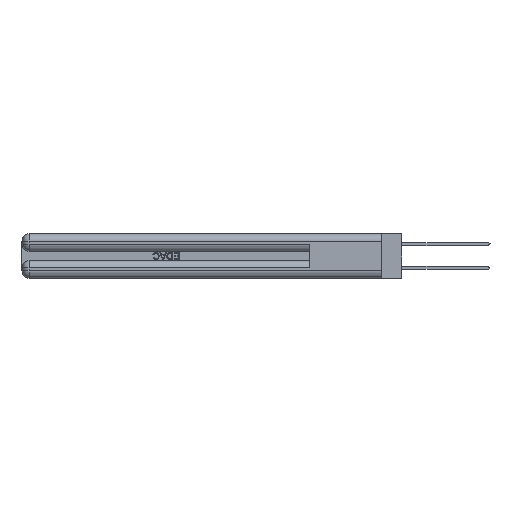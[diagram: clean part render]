
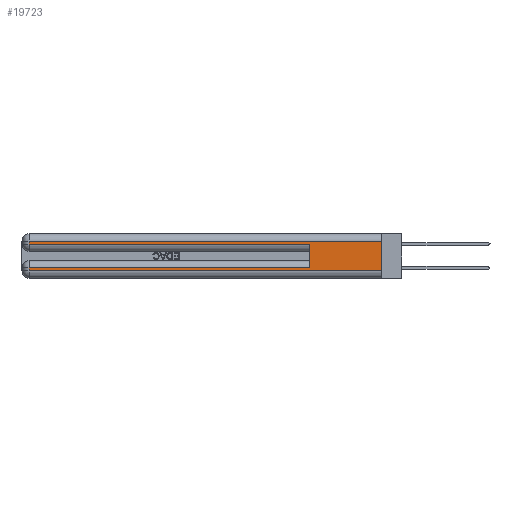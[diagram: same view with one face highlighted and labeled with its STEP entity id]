
A CAD part, left-side view. The second image highlights one B-rep face of the part: STEP entity #19723.
In plain terms, the highlighted planar face has unit normal (-1, 0, 0).
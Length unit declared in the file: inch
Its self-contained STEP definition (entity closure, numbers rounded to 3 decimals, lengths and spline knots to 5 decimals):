
#172 = EDGE_CURVE ( 'NONE', #41461, #45304, #2076, .T. ) ;
#293 = CARTESIAN_POINT ( 'NONE',  ( 0., 0., 0.085 ) ) ;
#947 = CARTESIAN_POINT ( 'NONE',  ( 0., 0., 0.37 ) ) ;
#2076 = LINE ( 'NONE', #7355, #39697 ) ;
#2754 = LINE ( 'NONE', #13703, #36304 ) ;
#3650 = LINE ( 'NONE', #4636, #18855 ) ;
#4143 = CARTESIAN_POINT ( 'NONE',  ( 0., 2.94, 0.31 ) ) ;
#4265 = CARTESIAN_POINT ( 'NONE',  ( 0., 2.94, 0.06 ) ) ;
#4636 = CARTESIAN_POINT ( 'NONE',  ( 0., 2.94, 0.37 ) ) ;
#5102 = CARTESIAN_POINT ( 'NONE',  ( 0., 0., 0.31 ) ) ;
#5394 = ORIENTED_EDGE ( 'NONE', *, *, #16337, .T. ) ;
#5699 = LINE ( 'NONE', #9321, #15059 ) ;
#6045 = DIRECTION ( 'NONE',  ( 0., -1., 0. ) ) ;
#6393 = PLANE ( 'NONE',  #37732 ) ;
#7355 = CARTESIAN_POINT ( 'NONE',  ( 0., 2.94, 0.37 ) ) ;
#8969 = VECTOR ( 'NONE', #22757, 39.37008 ) ;
#9321 = CARTESIAN_POINT ( 'NONE',  ( 0., 0., 0.06 ) ) ;
#10417 = EDGE_CURVE ( 'NONE', #42172, #28726, #33186, .T. ) ;
#11933 = VECTOR ( 'NONE', #39482, 39.37008 ) ;
#12002 = DIRECTION ( 'NONE',  ( 0., 0., -1. ) ) ;
#13620 = EDGE_CURVE ( 'NONE', #42172, #26062, #44048, .T. ) ;
#13703 = CARTESIAN_POINT ( 'NONE',  ( 0., 0.6, 0.145 ) ) ;
#15059 = VECTOR ( 'NONE', #6045, 39.37008 ) ;
#15963 = CARTESIAN_POINT ( 'NONE',  ( 0., 0.6, 0.085 ) ) ;
#16337 = EDGE_CURVE ( 'NONE', #29624, #45047, #26652, .T. ) ;
#16600 = CARTESIAN_POINT ( 'NONE',  ( 0., 0., 0.31 ) ) ;
#16651 = DIRECTION ( 'NONE',  ( 0., 0., -1. ) ) ;
#17339 = DIRECTION ( 'NONE',  ( 1., 0., 0. ) ) ;
#18855 = VECTOR ( 'NONE', #12002, 39.37008 ) ;
#19723 = ADVANCED_FACE ( 'NONE', ( #25156 ), #6393, .F. ) ;
#21315 = CARTESIAN_POINT ( 'NONE',  ( 0., 0., 0.37 ) ) ;
#21465 = ORIENTED_EDGE ( 'NONE', *, *, #13620, .T. ) ;
#22361 = EDGE_LOOP ( 'NONE', ( #28012, #21465, #35559, #5394, #24233, #41038, #42004, #28893 ) ) ;
#22757 = DIRECTION ( 'NONE',  ( 0., 1., 0. ) ) ;
#23134 = EDGE_CURVE ( 'NONE', #32164, #41461, #41915, .T. ) ;
#24019 = DIRECTION ( 'NONE',  ( 0., 1., 0. ) ) ;
#24233 = ORIENTED_EDGE ( 'NONE', *, *, #48264, .F. ) ;
#24328 = CARTESIAN_POINT ( 'NONE',  ( 0., 0., 0.285 ) ) ;
#25156 = FACE_OUTER_BOUND ( 'NONE', #22361, .T. ) ;
#26062 = VERTEX_POINT ( 'NONE', #4143 ) ;
#26652 = LINE ( 'NONE', #24328, #11933 ) ;
#28012 = ORIENTED_EDGE ( 'NONE', *, *, #10417, .F. ) ;
#28726 = VERTEX_POINT ( 'NONE', #34109 ) ;
#28893 = ORIENTED_EDGE ( 'NONE', *, *, #33861, .T. ) ;
#29624 = VERTEX_POINT ( 'NONE', #36515 ) ;
#32164 = VERTEX_POINT ( 'NONE', #15963 ) ;
#33186 = LINE ( 'NONE', #947, #37291 ) ;
#33861 = EDGE_CURVE ( 'NONE', #45304, #28726, #5699, .T. ) ;
#34030 = VECTOR ( 'NONE', #24019, 39.37008 ) ;
#34109 = CARTESIAN_POINT ( 'NONE',  ( 0., 0., 0.06 ) ) ;
#35553 = CARTESIAN_POINT ( 'NONE',  ( 0., 0.6, 0.285 ) ) ;
#35559 = ORIENTED_EDGE ( 'NONE', *, *, #44638, .T. ) ;
#36304 = VECTOR ( 'NONE', #39059, 39.37008 ) ;
#36326 = DIRECTION ( 'NONE',  ( 0., 0., -1. ) ) ;
#36515 = CARTESIAN_POINT ( 'NONE',  ( 0., 2.94, 0.285 ) ) ;
#37291 = VECTOR ( 'NONE', #16651, 39.37008 ) ;
#37732 = AXIS2_PLACEMENT_3D ( 'NONE', #21315, #17339, #36326 ) ;
#39059 = DIRECTION ( 'NONE',  ( 0., 0., 1. ) ) ;
#39482 = DIRECTION ( 'NONE',  ( 0., -1., 0. ) ) ;
#39697 = VECTOR ( 'NONE', #48184, 39.37008 ) ;
#41038 = ORIENTED_EDGE ( 'NONE', *, *, #23134, .T. ) ;
#41461 = VERTEX_POINT ( 'NONE', #46105 ) ;
#41915 = LINE ( 'NONE', #293, #8969 ) ;
#42004 = ORIENTED_EDGE ( 'NONE', *, *, #172, .T. ) ;
#42172 = VERTEX_POINT ( 'NONE', #5102 ) ;
#44048 = LINE ( 'NONE', #16600, #34030 ) ;
#44638 = EDGE_CURVE ( 'NONE', #26062, #29624, #3650, .T. ) ;
#45047 = VERTEX_POINT ( 'NONE', #35553 ) ;
#45304 = VERTEX_POINT ( 'NONE', #4265 ) ;
#46105 = CARTESIAN_POINT ( 'NONE',  ( 0., 2.94, 0.085 ) ) ;
#48184 = DIRECTION ( 'NONE',  ( 0., 0., -1. ) ) ;
#48264 = EDGE_CURVE ( 'NONE', #32164, #45047, #2754, .T. ) ;
